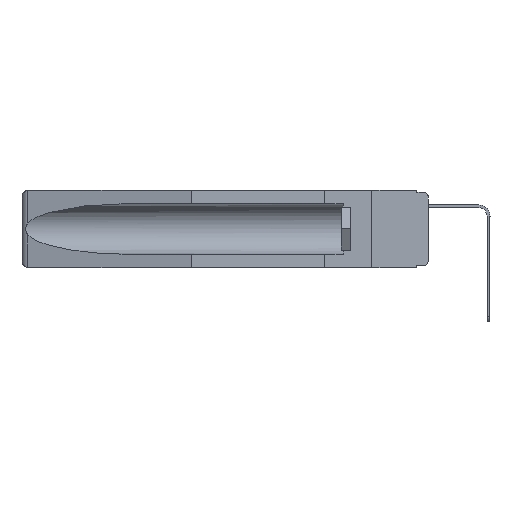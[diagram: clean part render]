
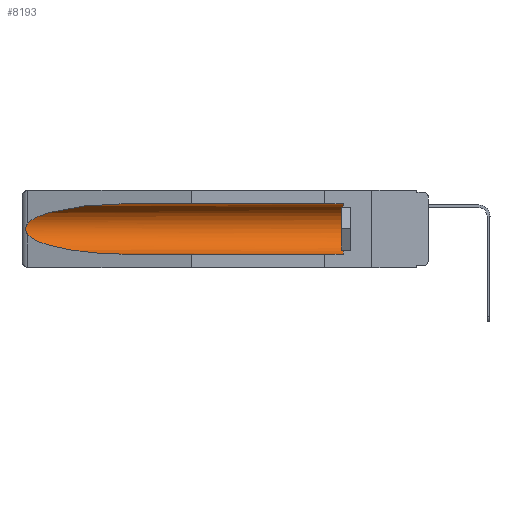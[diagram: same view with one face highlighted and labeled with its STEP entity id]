
A CAD part, left-side view. The second image highlights one B-rep face of the part: STEP entity #8193.
In plain terms, the highlighted cylindrical face has radius 2.857 mm (diameter 5.715 mm), a partial arc.
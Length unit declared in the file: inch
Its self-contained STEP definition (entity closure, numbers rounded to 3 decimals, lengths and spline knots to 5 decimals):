
#546 = DIRECTION ( 'NONE',  ( 0., 0., 1. ) ) ;
#590 = CARTESIAN_POINT ( 'NONE',  ( 0.2673, 1.5327, -0.16383 ) ) ;
#720 = CARTESIAN_POINT ( 'NONE',  ( 0.26537, 1.52718, -0.19328 ) ) ;
#802 = DIRECTION ( 'NONE',  ( 0., 1., 0. ) ) ;
#1149 = ORIENTED_EDGE ( 'NONE', *, *, #12721, .F. ) ;
#1159 = LINE ( 'NONE', #3610, #1403 ) ;
#1392 = EDGE_CURVE ( 'NONE', #14646, #6454, #1159, .T. ) ;
#1403 = VECTOR ( 'NONE', #18535, 39.37008 ) ;
#1758 = CARTESIAN_POINT ( 'NONE',  ( 0.26537, 1.52718, -0.14972 ) ) ;
#1886 = CARTESIAN_POINT ( 'NONE',  ( 0.25451, 1.48313, -0.09465 ) ) ;
#2066 = VECTOR ( 'NONE', #10606, 39.37008 ) ;
#2909 = EDGE_CURVE ( 'NONE', #10185, #8670, #8933, .T. ) ;
#3137 = CARTESIAN_POINT ( 'NONE',  ( 0.26537, 1.52718, -0.14972 ) ) ;
#3569 = ORIENTED_EDGE ( 'NONE', *, *, #2909, .T. ) ;
#3610 = CARTESIAN_POINT ( 'NONE',  ( 0.155, -0.30754, -0.059 ) ) ;
#3623 = EDGE_LOOP ( 'NONE', ( #8332, #10757, #3569, #1149, #16478, #14393 ) ) ;
#3765 = CARTESIAN_POINT ( 'NONE',  ( 0.2675, 1.53308, -0.16763 ) ) ;
#4522 = CARTESIAN_POINT ( 'NONE',  ( 0.26537, 1.52718, -0.19328 ) ) ;
#4734 = CARTESIAN_POINT ( 'NONE',  ( 0.21114, 1.30732, -0.059 ) ) ;
#5016 = CARTESIAN_POINT ( 'NONE',  ( 0.26537, 1.52718, -0.14972 ) ) ;
#5076 = CARTESIAN_POINT ( 'NONE',  ( 0.2675, 1.53308, -0.17534 ) ) ;
#5131 = LINE ( 'NONE', #6047, #2066 ) ;
#5161 = CARTESIAN_POINT ( 'NONE',  ( 0.155, -0.30754, -0.1715 ) ) ;
#5489 =( BOUNDED_CURVE ( )  B_SPLINE_CURVE ( 3, ( #13693, #4734, #1886, #1758 ),
 .UNSPECIFIED., .F., .F. ) 
 B_SPLINE_CURVE_WITH_KNOTS ( ( 4, 4 ),
 ( 4.71239, 6.08839 ),
 .UNSPECIFIED. ) 
 CURVE ( )  GEOMETRIC_REPRESENTATION_ITEM ( )  RATIONAL_B_SPLINE_CURVE ( ( 1., 0.848, 0.848, 1. ) ) 
 REPRESENTATION_ITEM ( '' )  );
#6047 = CARTESIAN_POINT ( 'NONE',  ( 0.155, -0.30754, -0.284 ) ) ;
#6076 = VERTEX_POINT ( 'NONE', #3137 ) ;
#6240 = CARTESIAN_POINT ( 'NONE',  ( 0.155, 0.126, -0.059 ) ) ;
#6258 = FACE_OUTER_BOUND ( 'NONE', #3623, .T. ) ;
#6454 = VERTEX_POINT ( 'NONE', #15712 ) ;
#6571 = CARTESIAN_POINT ( 'NONE',  ( 0.26597, 1.5296, -0.19026 ) ) ;
#6582 = EDGE_CURVE ( 'NONE', #6076, #10185, #17430, .T. ) ;
#7674 = EDGE_CURVE ( 'NONE', #14967, #14646, #10248, .T. ) ;
#8193 = ADVANCED_FACE ( 'NONE', ( #6258 ), #11623, .F. ) ;
#8332 = ORIENTED_EDGE ( 'NONE', *, *, #11476, .T. ) ;
#8670 = VERTEX_POINT ( 'NONE', #11374 ) ;
#8933 =( BOUNDED_CURVE ( )  B_SPLINE_CURVE ( 3, ( #18324, #16638, #9194, #12163 ),
 .UNSPECIFIED., .F., .F. ) 
 B_SPLINE_CURVE_WITH_KNOTS ( ( 4, 4 ),
 ( 0.1948, 1.5708 ),
 .UNSPECIFIED. ) 
 CURVE ( )  GEOMETRIC_REPRESENTATION_ITEM ( )  RATIONAL_B_SPLINE_CURVE ( ( 1., 0.848, 0.848, 1. ) ) 
 REPRESENTATION_ITEM ( '' )  );
#9194 = CARTESIAN_POINT ( 'NONE',  ( 0.21114, 1.30732, -0.284 ) ) ;
#9260 = CARTESIAN_POINT ( 'NONE',  ( 0.155, 0.126, -0.1715 ) ) ;
#9391 = DIRECTION ( 'NONE',  ( 0., 0., 1. ) ) ;
#10185 = VERTEX_POINT ( 'NONE', #4522 ) ;
#10248 = CIRCLE ( 'NONE', #15761, 0.1125 ) ;
#10427 = CARTESIAN_POINT ( 'NONE',  ( 0.155, 0.126, -0.284 ) ) ;
#10606 = DIRECTION ( 'NONE',  ( 0., 1., 0. ) ) ;
#10757 = ORIENTED_EDGE ( 'NONE', *, *, #6582, .T. ) ;
#11374 = CARTESIAN_POINT ( 'NONE',  ( 0.155, 1.07973, -0.284 ) ) ;
#11476 = EDGE_CURVE ( 'NONE', #6454, #6076, #5489, .T. ) ;
#11623 = CYLINDRICAL_SURFACE ( 'NONE', #12090, 0.1125 ) ;
#12090 = AXIS2_PLACEMENT_3D ( 'NONE', #5161, #802, #546 ) ;
#12163 = CARTESIAN_POINT ( 'NONE',  ( 0.155, 1.07973, -0.284 ) ) ;
#12532 = CARTESIAN_POINT ( 'NONE',  ( 0.26655, 1.53094, -0.18657 ) ) ;
#12721 = EDGE_CURVE ( 'NONE', #14967, #8670, #5131, .T. ) ;
#13693 = CARTESIAN_POINT ( 'NONE',  ( 0.155, 1.07973, -0.059 ) ) ;
#13745 = DIRECTION ( 'NONE',  ( 0., -1., 0. ) ) ;
#14123 = CARTESIAN_POINT ( 'NONE',  ( 0.26654, 1.53092, -0.15636 ) ) ;
#14393 = ORIENTED_EDGE ( 'NONE', *, *, #1392, .T. ) ;
#14646 = VERTEX_POINT ( 'NONE', #6240 ) ;
#14967 = VERTEX_POINT ( 'NONE', #10427 ) ;
#15574 = CARTESIAN_POINT ( 'NONE',  ( 0.2673, 1.53269, -0.17917 ) ) ;
#15712 = CARTESIAN_POINT ( 'NONE',  ( 0.155, 1.07973, -0.059 ) ) ;
#15761 = AXIS2_PLACEMENT_3D ( 'NONE', #9260, #13745, #9391 ) ;
#16478 = ORIENTED_EDGE ( 'NONE', *, *, #7674, .T. ) ;
#16638 = CARTESIAN_POINT ( 'NONE',  ( 0.25451, 1.48313, -0.24835 ) ) ;
#17430 = B_SPLINE_CURVE_WITH_KNOTS ( 'NONE', 3,
 ( #5016, #18498, #14123, #590, #3765, #5076, #15574, #12532, #6571, #720 ),
 .UNSPECIFIED., .F., .F.,
 ( 4, 2, 2, 2, 4 ),
 ( 0., 0.00029, 0.00058, 0.00087, 0.00117 ),
 .UNSPECIFIED. ) ;
#18324 = CARTESIAN_POINT ( 'NONE',  ( 0.26537, 1.52718, -0.19328 ) ) ;
#18498 = CARTESIAN_POINT ( 'NONE',  ( 0.26597, 1.52961, -0.15275 ) ) ;
#18535 = DIRECTION ( 'NONE',  ( 0., 1., 0. ) ) ;
